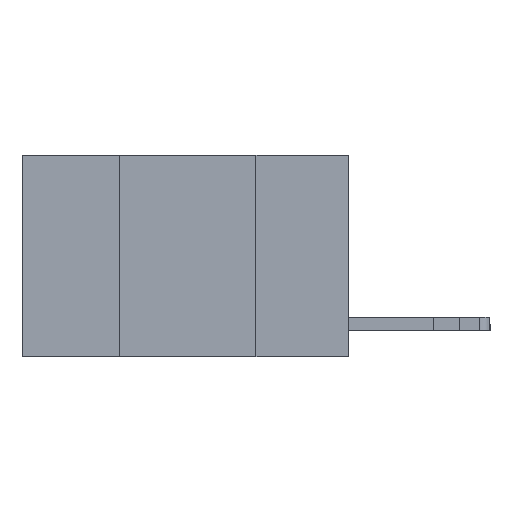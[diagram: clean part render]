
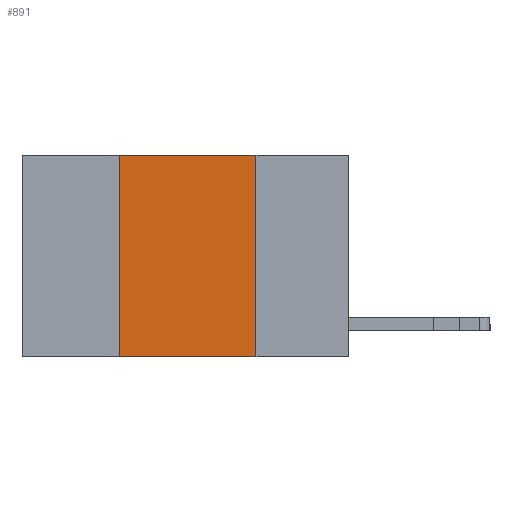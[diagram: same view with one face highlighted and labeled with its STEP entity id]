
A CAD part, left-side view. The second image highlights one B-rep face of the part: STEP entity #891.
In plain terms, the highlighted planar face has unit normal (-1, 0, 0).
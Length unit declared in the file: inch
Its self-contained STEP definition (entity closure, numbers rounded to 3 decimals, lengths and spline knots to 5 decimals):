
#685 = VERTEX_POINT ( 'NONE', #2697 ) ;
#891 = ADVANCED_FACE ( 'NONE', ( #10846 ), #2125, .F. ) ;
#1303 = AXIS2_PLACEMENT_3D ( 'NONE', #11889, #3492, #3574 ) ;
#1345 = CARTESIAN_POINT ( 'NONE',  ( 0., 0.6, 0. ) ) ;
#1349 = DIRECTION ( 'NONE',  ( 0., 0., -1. ) ) ;
#2101 = LINE ( 'NONE', #7010, #15237 ) ;
#2125 = PLANE ( 'NONE',  #1303 ) ;
#2401 = LINE ( 'NONE', #1345, #8505 ) ;
#2697 = CARTESIAN_POINT ( 'NONE',  ( 0., 0.42, 0. ) ) ;
#3341 = CARTESIAN_POINT ( 'NONE',  ( 0., 0.42, -0.37 ) ) ;
#3357 = CARTESIAN_POINT ( 'NONE',  ( 0., 0.42, 0. ) ) ;
#3492 = DIRECTION ( 'NONE',  ( 1., 0., 0. ) ) ;
#3574 = DIRECTION ( 'NONE',  ( 0., 0., -1. ) ) ;
#4669 = ORIENTED_EDGE ( 'NONE', *, *, #15480, .F. ) ;
#5101 = EDGE_CURVE ( 'NONE', #685, #9778, #2401, .T. ) ;
#5330 = DIRECTION ( 'NONE',  ( 0., 0., 1. ) ) ;
#6017 = DIRECTION ( 'NONE',  ( 0., -1., 0. ) ) ;
#6259 = CARTESIAN_POINT ( 'NONE',  ( 0., 0.17, 0. ) ) ;
#6987 = LINE ( 'NONE', #3357, #14098 ) ;
#7010 = CARTESIAN_POINT ( 'NONE',  ( 0., 0.6, -0.37 ) ) ;
#7325 = LINE ( 'NONE', #6259, #13426 ) ;
#7710 = EDGE_CURVE ( 'NONE', #9778, #13847, #7325, .T. ) ;
#7771 = CARTESIAN_POINT ( 'NONE',  ( 0., 0.17, 0. ) ) ;
#8505 = VECTOR ( 'NONE', #6017, 39.37008 ) ;
#8605 = EDGE_CURVE ( 'NONE', #9625, #13847, #2101, .T. ) ;
#9595 = EDGE_LOOP ( 'NONE', ( #14089, #14552, #4669, #14391 ) ) ;
#9625 = VERTEX_POINT ( 'NONE', #3341 ) ;
#9778 = VERTEX_POINT ( 'NONE', #7771 ) ;
#10816 = DIRECTION ( 'NONE',  ( 0., -1., 0. ) ) ;
#10846 = FACE_OUTER_BOUND ( 'NONE', #9595, .T. ) ;
#11889 = CARTESIAN_POINT ( 'NONE',  ( 0., 0.6, 0. ) ) ;
#13426 = VECTOR ( 'NONE', #1349, 39.37008 ) ;
#13847 = VERTEX_POINT ( 'NONE', #14832 ) ;
#14089 = ORIENTED_EDGE ( 'NONE', *, *, #7710, .F. ) ;
#14098 = VECTOR ( 'NONE', #5330, 39.37008 ) ;
#14391 = ORIENTED_EDGE ( 'NONE', *, *, #8605, .T. ) ;
#14552 = ORIENTED_EDGE ( 'NONE', *, *, #5101, .F. ) ;
#14832 = CARTESIAN_POINT ( 'NONE',  ( 0., 0.17, -0.37 ) ) ;
#15237 = VECTOR ( 'NONE', #10816, 39.37008 ) ;
#15480 = EDGE_CURVE ( 'NONE', #9625, #685, #6987, .T. ) ;
